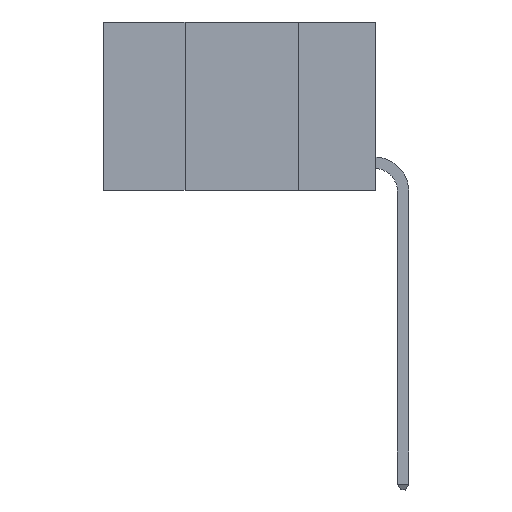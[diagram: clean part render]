
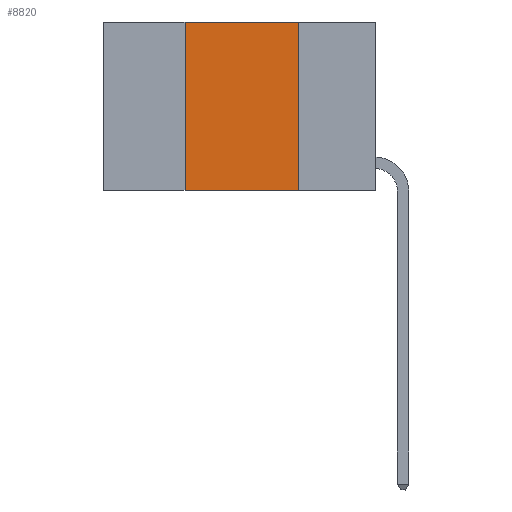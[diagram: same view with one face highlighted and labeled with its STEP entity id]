
A CAD part, left-side view. The second image highlights one B-rep face of the part: STEP entity #8820.
In plain terms, the highlighted planar face has unit normal (-1, 0, 0).
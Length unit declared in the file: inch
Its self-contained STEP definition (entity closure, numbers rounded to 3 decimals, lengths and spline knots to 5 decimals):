
#753 = EDGE_CURVE ( 'NONE', #23698, #964, #23420, .T. ) ;
#964 = VERTEX_POINT ( 'NONE', #12207 ) ;
#2728 = CARTESIAN_POINT ( 'NONE',  ( 0., 0.17, 0. ) ) ;
#2978 = VECTOR ( 'NONE', #22241, 39.37008 ) ;
#3816 = VECTOR ( 'NONE', #20492, 39.37008 ) ;
#3903 = CARTESIAN_POINT ( 'NONE',  ( 0., 0.6, 0. ) ) ;
#4229 = ORIENTED_EDGE ( 'NONE', *, *, #19879, .F. ) ;
#6205 = CARTESIAN_POINT ( 'NONE',  ( 0., 0.17, 0. ) ) ;
#6229 = PLANE ( 'NONE',  #22622 ) ;
#7175 = LINE ( 'NONE', #26971, #24739 ) ;
#7864 = CARTESIAN_POINT ( 'NONE',  ( 0., 0.42, -0.37 ) ) ;
#8542 = DIRECTION ( 'NONE',  ( 1., 0., 0. ) ) ;
#8820 = ADVANCED_FACE ( 'NONE', ( #26182 ), #6229, .F. ) ;
#9042 = CARTESIAN_POINT ( 'NONE',  ( 0., 0.6, 0. ) ) ;
#12097 = VERTEX_POINT ( 'NONE', #2728 ) ;
#12207 = CARTESIAN_POINT ( 'NONE',  ( 0., 0.17, -0.37 ) ) ;
#13288 = ORIENTED_EDGE ( 'NONE', *, *, #753, .T. ) ;
#13561 = DIRECTION ( 'NONE',  ( 0., 0., 1. ) ) ;
#14950 = VERTEX_POINT ( 'NONE', #19045 ) ;
#15271 = LINE ( 'NONE', #6205, #2978 ) ;
#17355 = VECTOR ( 'NONE', #29373, 39.37008 ) ;
#17928 = ORIENTED_EDGE ( 'NONE', *, *, #22469, .F. ) ;
#18458 = EDGE_LOOP ( 'NONE', ( #4229, #29294, #17928, #13288 ) ) ;
#19045 = CARTESIAN_POINT ( 'NONE',  ( 0., 0.42, 0. ) ) ;
#19879 = EDGE_CURVE ( 'NONE', #12097, #964, #15271, .T. ) ;
#20492 = DIRECTION ( 'NONE',  ( 0., -1., 0. ) ) ;
#21417 = LINE ( 'NONE', #9042, #3816 ) ;
#22241 = DIRECTION ( 'NONE',  ( 0., 0., -1. ) ) ;
#22469 = EDGE_CURVE ( 'NONE', #23698, #14950, #7175, .T. ) ;
#22622 = AXIS2_PLACEMENT_3D ( 'NONE', #3903, #8542, #24565 ) ;
#23420 = LINE ( 'NONE', #25402, #17355 ) ;
#23698 = VERTEX_POINT ( 'NONE', #7864 ) ;
#24016 = EDGE_CURVE ( 'NONE', #14950, #12097, #21417, .T. ) ;
#24565 = DIRECTION ( 'NONE',  ( 0., 0., -1. ) ) ;
#24739 = VECTOR ( 'NONE', #13561, 39.37008 ) ;
#25402 = CARTESIAN_POINT ( 'NONE',  ( 0., 0.6, -0.37 ) ) ;
#26182 = FACE_OUTER_BOUND ( 'NONE', #18458, .T. ) ;
#26971 = CARTESIAN_POINT ( 'NONE',  ( 0., 0.42, 0. ) ) ;
#29294 = ORIENTED_EDGE ( 'NONE', *, *, #24016, .F. ) ;
#29373 = DIRECTION ( 'NONE',  ( 0., -1., 0. ) ) ;
